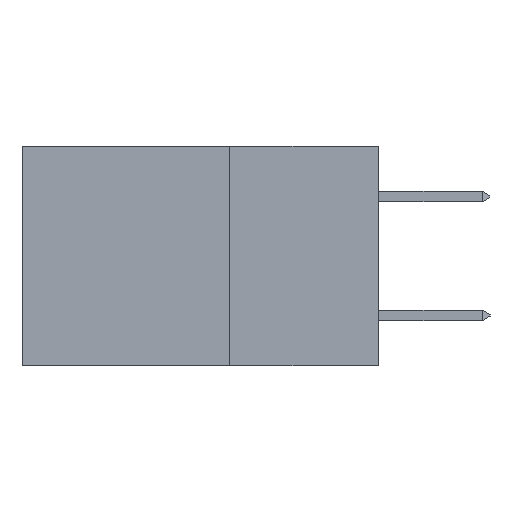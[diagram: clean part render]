
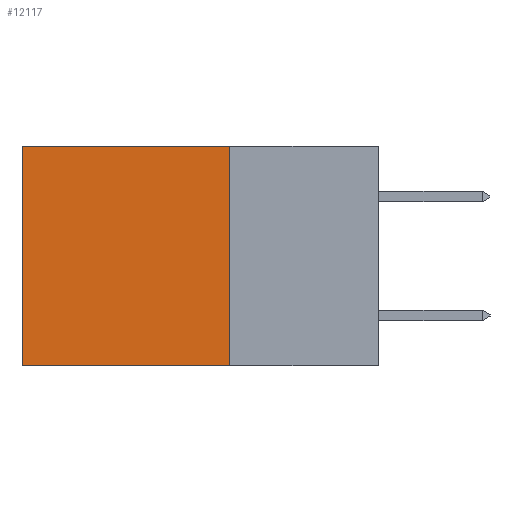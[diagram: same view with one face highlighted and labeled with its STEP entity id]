
A CAD part, left-side view. The second image highlights one B-rep face of the part: STEP entity #12117.
In plain terms, the highlighted planar face has unit normal (-1, 0, 0).
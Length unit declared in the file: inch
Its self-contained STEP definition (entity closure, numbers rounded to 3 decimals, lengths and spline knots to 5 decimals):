
#780 = LINE ( 'NONE', #10444, #8858 ) ;
#841 = VECTOR ( 'NONE', #13812, 39.37008 ) ;
#2464 = DIRECTION ( 'NONE',  ( 0., 0., -1. ) ) ;
#2646 = VECTOR ( 'NONE', #4858, 39.37008 ) ;
#3026 = VERTEX_POINT ( 'NONE', #15944 ) ;
#3169 = LINE ( 'NONE', #13340, #2646 ) ;
#3344 = DIRECTION ( 'NONE',  ( 0., 1., 0. ) ) ;
#3497 = CARTESIAN_POINT ( 'NONE',  ( 0.2615, 0.25, -0.37 ) ) ;
#4313 = LINE ( 'NONE', #3497, #17338 ) ;
#4858 = DIRECTION ( 'NONE',  ( 0., 0., -1. ) ) ;
#4888 = ORIENTED_EDGE ( 'NONE', *, *, #14968, .F. ) ;
#5669 = CARTESIAN_POINT ( 'NONE',  ( 0.2615, 0.6, -0.37 ) ) ;
#7388 = VERTEX_POINT ( 'NONE', #5669 ) ;
#7602 = EDGE_CURVE ( 'NONE', #16337, #10080, #14489, .T. ) ;
#8540 = EDGE_CURVE ( 'NONE', #3026, #7388, #4313, .T. ) ;
#8858 = VECTOR ( 'NONE', #8934, 39.37008 ) ;
#8934 = DIRECTION ( 'NONE',  ( 0., 0., -1. ) ) ;
#8990 = EDGE_CURVE ( 'NONE', #10080, #7388, #780, .T. ) ;
#10080 = VERTEX_POINT ( 'NONE', #17448 ) ;
#10444 = CARTESIAN_POINT ( 'NONE',  ( 0.2615, 0.6, -0.37 ) ) ;
#11007 = CARTESIAN_POINT ( 'NONE',  ( 0.2615, 0.25, 0. ) ) ;
#11027 = CARTESIAN_POINT ( 'NONE',  ( 0.2615, 0.25, -0.37 ) ) ;
#11798 = EDGE_LOOP ( 'NONE', ( #16173, #14478, #4888, #16379 ) ) ;
#12117 = ADVANCED_FACE ( 'NONE', ( #15062 ), #17734, .F. ) ;
#12702 = DIRECTION ( 'NONE',  ( 1., 0., 0. ) ) ;
#13340 = CARTESIAN_POINT ( 'NONE',  ( 0.2615, 0.25, -0.37 ) ) ;
#13812 = DIRECTION ( 'NONE',  ( 0., 1., 0. ) ) ;
#13868 = CARTESIAN_POINT ( 'NONE',  ( 0.2615, 0.25, 0. ) ) ;
#14478 = ORIENTED_EDGE ( 'NONE', *, *, #8540, .F. ) ;
#14489 = LINE ( 'NONE', #13868, #841 ) ;
#14968 = EDGE_CURVE ( 'NONE', #16337, #3026, #3169, .T. ) ;
#15062 = FACE_OUTER_BOUND ( 'NONE', #11798, .T. ) ;
#15944 = CARTESIAN_POINT ( 'NONE',  ( 0.2615, 0.25, -0.37 ) ) ;
#16173 = ORIENTED_EDGE ( 'NONE', *, *, #8990, .T. ) ;
#16337 = VERTEX_POINT ( 'NONE', #11007 ) ;
#16379 = ORIENTED_EDGE ( 'NONE', *, *, #7602, .T. ) ;
#17175 = AXIS2_PLACEMENT_3D ( 'NONE', #11027, #12702, #2464 ) ;
#17338 = VECTOR ( 'NONE', #3344, 39.37008 ) ;
#17448 = CARTESIAN_POINT ( 'NONE',  ( 0.2615, 0.6, 0. ) ) ;
#17734 = PLANE ( 'NONE',  #17175 ) ;
